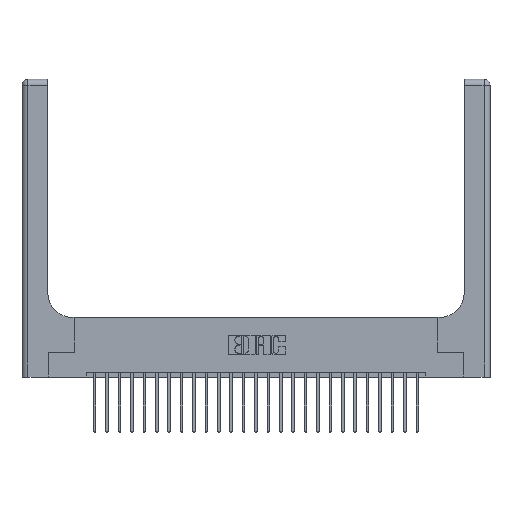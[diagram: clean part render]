
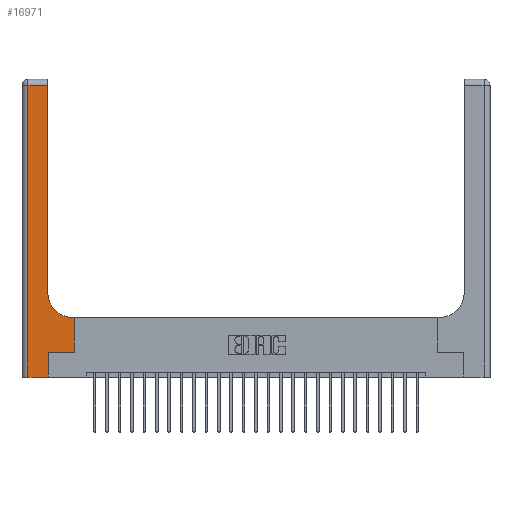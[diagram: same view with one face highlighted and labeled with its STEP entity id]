
A CAD part, top view. The second image highlights one B-rep face of the part: STEP entity #16971.
In plain terms, the highlighted planar face has unit normal (0, 0, 1).
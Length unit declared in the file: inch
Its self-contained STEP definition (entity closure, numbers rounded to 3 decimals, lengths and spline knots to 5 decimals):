
#365 = EDGE_CURVE ( 'NONE', #13882, #4428, #1851, .T. ) ;
#609 = DIRECTION ( 'NONE',  ( -1., 0., 0. ) ) ;
#808 = ORIENTED_EDGE ( 'NONE', *, *, #17852, .T. ) ;
#840 = AXIS2_PLACEMENT_3D ( 'NONE', #3346, #14719, #22520 ) ;
#962 = VERTEX_POINT ( 'NONE', #9962 ) ;
#1205 = FACE_OUTER_BOUND ( 'NONE', #21923, .T. ) ;
#1436 = ORIENTED_EDGE ( 'NONE', *, *, #4949, .T. ) ;
#1447 = CARTESIAN_POINT ( 'NONE',  ( 0.06, 3., 0.37 ) ) ;
#1812 = VECTOR ( 'NONE', #17299, 39.37008 ) ;
#1851 = LINE ( 'NONE', #19323, #9832 ) ;
#2086 = EDGE_CURVE ( 'NONE', #2788, #13882, #9121, .T. ) ;
#2354 = VERTEX_POINT ( 'NONE', #16650 ) ;
#2639 = CARTESIAN_POINT ( 'NONE',  ( 0.06, 0., 0.37 ) ) ;
#2788 = VERTEX_POINT ( 'NONE', #4955 ) ;
#3346 = CARTESIAN_POINT ( 'NONE',  ( 0.51, 0.85, 0.37 ) ) ;
#3700 = DIRECTION ( 'NONE',  ( 0., 1., 0. ) ) ;
#3758 = LINE ( 'NONE', #25277, #17406 ) ;
#3975 = EDGE_CURVE ( 'NONE', #4428, #18740, #13411, .T. ) ;
#4424 = LINE ( 'NONE', #12332, #6931 ) ;
#4428 = VERTEX_POINT ( 'NONE', #11448 ) ;
#4949 = EDGE_CURVE ( 'NONE', #23787, #2788, #3758, .T. ) ;
#4955 = CARTESIAN_POINT ( 'NONE',  ( 0.265, 0., 0.37 ) ) ;
#5050 = VECTOR ( 'NONE', #24773, 39.37008 ) ;
#5059 = VECTOR ( 'NONE', #23272, 39.37008 ) ;
#5466 = DIRECTION ( 'NONE',  ( 0., 1., 0. ) ) ;
#5811 = EDGE_CURVE ( 'NONE', #18262, #962, #4424, .T. ) ;
#6916 = EDGE_CURVE ( 'NONE', #2354, #9397, #11831, .T. ) ;
#6931 = VECTOR ( 'NONE', #609, 39.37008 ) ;
#6961 = VECTOR ( 'NONE', #5466, 39.37008 ) ;
#7438 = LINE ( 'NONE', #15149, #1812 ) ;
#9121 = LINE ( 'NONE', #20869, #5050 ) ;
#9397 = VERTEX_POINT ( 'NONE', #18110 ) ;
#9583 = LINE ( 'NONE', #1447, #5059 ) ;
#9620 = DIRECTION ( 'NONE',  ( 1., 0., 0. ) ) ;
#9832 = VECTOR ( 'NONE', #9620, 39.37008 ) ;
#9962 = CARTESIAN_POINT ( 'NONE',  ( 0.06, 2.94, 0.37 ) ) ;
#10004 = ORIENTED_EDGE ( 'NONE', *, *, #10059, .T. ) ;
#10059 = EDGE_CURVE ( 'NONE', #18740, #2354, #7438, .T. ) ;
#10650 = ORIENTED_EDGE ( 'NONE', *, *, #365, .T. ) ;
#10775 = DIRECTION ( 'NONE',  ( -1., 0., 0. ) ) ;
#10915 = DIRECTION ( 'NONE',  ( 0., 0., -1. ) ) ;
#10917 = CARTESIAN_POINT ( 'NONE',  ( 0.265, 0.25, 0.37 ) ) ;
#11448 = CARTESIAN_POINT ( 'NONE',  ( 0.528, 0.25, 0.37 ) ) ;
#11831 = CIRCLE ( 'NONE', #840, 0.25 ) ;
#12332 = CARTESIAN_POINT ( 'NONE',  ( 0., 2.94, 0.37 ) ) ;
#12411 = ORIENTED_EDGE ( 'NONE', *, *, #6916, .T. ) ;
#13411 = LINE ( 'NONE', #21201, #14937 ) ;
#13664 = ORIENTED_EDGE ( 'NONE', *, *, #2086, .T. ) ;
#13882 = VERTEX_POINT ( 'NONE', #10917 ) ;
#14597 = AXIS2_PLACEMENT_3D ( 'NONE', #24100, #10915, #10775 ) ;
#14719 = DIRECTION ( 'NONE',  ( 0., 0., -1. ) ) ;
#14937 = VECTOR ( 'NONE', #3700, 39.37008 ) ;
#15149 = CARTESIAN_POINT ( 'NONE',  ( 0.26, 0.6, 0.37 ) ) ;
#15189 = LINE ( 'NONE', #15449, #6961 ) ;
#15449 = CARTESIAN_POINT ( 'NONE',  ( 0.26, 3., 0.37 ) ) ;
#16650 = CARTESIAN_POINT ( 'NONE',  ( 0.51, 0.6, 0.37 ) ) ;
#16971 = ADVANCED_FACE ( 'NONE', ( #1205 ), #24604, .F. ) ;
#17299 = DIRECTION ( 'NONE',  ( -1., 0., 0. ) ) ;
#17406 = VECTOR ( 'NONE', #25148, 39.37008 ) ;
#17852 = EDGE_CURVE ( 'NONE', #962, #23787, #9583, .T. ) ;
#18110 = CARTESIAN_POINT ( 'NONE',  ( 0.26, 0.85, 0.37 ) ) ;
#18262 = VERTEX_POINT ( 'NONE', #19151 ) ;
#18740 = VERTEX_POINT ( 'NONE', #22941 ) ;
#19151 = CARTESIAN_POINT ( 'NONE',  ( 0.26, 2.94, 0.37 ) ) ;
#19323 = CARTESIAN_POINT ( 'NONE',  ( 0.265, 0.25, 0.37 ) ) ;
#20827 = ORIENTED_EDGE ( 'NONE', *, *, #5811, .T. ) ;
#20869 = CARTESIAN_POINT ( 'NONE',  ( 0.265, 0., 0.37 ) ) ;
#21201 = CARTESIAN_POINT ( 'NONE',  ( 0.528, 0.25, 0.37 ) ) ;
#21335 = ORIENTED_EDGE ( 'NONE', *, *, #3975, .T. ) ;
#21923 = EDGE_LOOP ( 'NONE', ( #24297, #20827, #808, #1436, #13664, #10650, #21335, #10004, #12411 ) ) ;
#22183 = EDGE_CURVE ( 'NONE', #9397, #18262, #15189, .T. ) ;
#22520 = DIRECTION ( 'NONE',  ( 1., 0., 0. ) ) ;
#22941 = CARTESIAN_POINT ( 'NONE',  ( 0.528, 0.6, 0.37 ) ) ;
#23272 = DIRECTION ( 'NONE',  ( 0., -1., 0. ) ) ;
#23787 = VERTEX_POINT ( 'NONE', #2639 ) ;
#24100 = CARTESIAN_POINT ( 'NONE',  ( 0., 3., 0.37 ) ) ;
#24297 = ORIENTED_EDGE ( 'NONE', *, *, #22183, .T. ) ;
#24604 = PLANE ( 'NONE',  #14597 ) ;
#24773 = DIRECTION ( 'NONE',  ( 0., 1., 0. ) ) ;
#25148 = DIRECTION ( 'NONE',  ( 1., 0., 0. ) ) ;
#25277 = CARTESIAN_POINT ( 'NONE',  ( 0., 0., 0.37 ) ) ;
